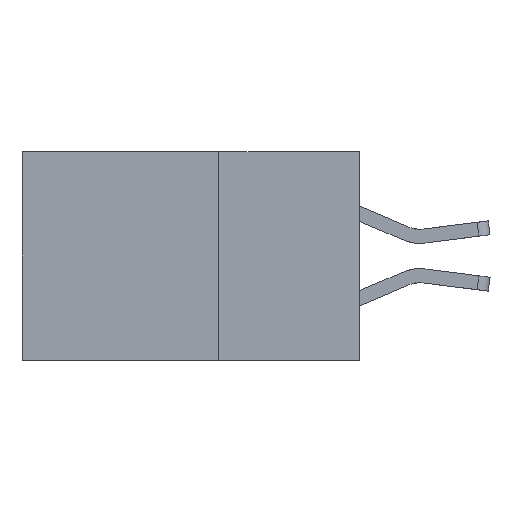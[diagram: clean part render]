
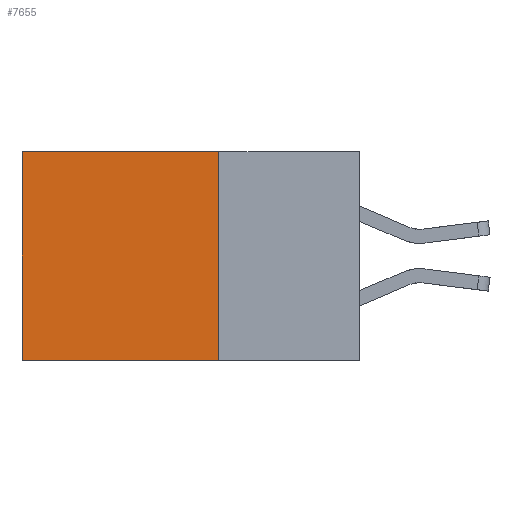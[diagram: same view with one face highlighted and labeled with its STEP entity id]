
A CAD part, left-side view. The second image highlights one B-rep face of the part: STEP entity #7655.
In plain terms, the highlighted planar face has unit normal (-1, 0, 0).
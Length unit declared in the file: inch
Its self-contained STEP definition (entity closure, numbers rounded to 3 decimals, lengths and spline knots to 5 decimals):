
#774 = VECTOR ( 'NONE', #14064, 39.37008 ) ;
#1554 = ORIENTED_EDGE ( 'NONE', *, *, #13683, .T. ) ;
#1603 = CARTESIAN_POINT ( 'NONE',  ( 0.2875, 0.25, 0. ) ) ;
#2073 = VERTEX_POINT ( 'NONE', #15092 ) ;
#2474 = EDGE_LOOP ( 'NONE', ( #10835, #10381, #4373, #1554 ) ) ;
#2613 = EDGE_CURVE ( 'NONE', #10566, #2073, #10315, .T. ) ;
#3414 = FACE_OUTER_BOUND ( 'NONE', #2474, .T. ) ;
#3689 = PLANE ( 'NONE',  #7501 ) ;
#4159 = DIRECTION ( 'NONE',  ( 0., 1., 0. ) ) ;
#4251 = CARTESIAN_POINT ( 'NONE',  ( 0.2875, 0.6, 0. ) ) ;
#4373 = ORIENTED_EDGE ( 'NONE', *, *, #2613, .F. ) ;
#4667 = CARTESIAN_POINT ( 'NONE',  ( 0.2875, 0.25, 0. ) ) ;
#4689 = CARTESIAN_POINT ( 'NONE',  ( 0.2875, 0.25, 0. ) ) ;
#4812 = VERTEX_POINT ( 'NONE', #14345 ) ;
#4959 = VERTEX_POINT ( 'NONE', #4251 ) ;
#6323 = VECTOR ( 'NONE', #14890, 39.37008 ) ;
#6869 = LINE ( 'NONE', #15251, #774 ) ;
#7501 = AXIS2_PLACEMENT_3D ( 'NONE', #4689, #13349, #9535 ) ;
#7655 = ADVANCED_FACE ( 'NONE', ( #3414 ), #3689, .F. ) ;
#8329 = VECTOR ( 'NONE', #14919, 39.37008 ) ;
#9535 = DIRECTION ( 'NONE',  ( 0., 0., -1. ) ) ;
#9717 = VECTOR ( 'NONE', #4159, 39.37008 ) ;
#10255 = EDGE_CURVE ( 'NONE', #2073, #4812, #11887, .T. ) ;
#10315 = LINE ( 'NONE', #1603, #6323 ) ;
#10381 = ORIENTED_EDGE ( 'NONE', *, *, #10255, .F. ) ;
#10566 = VERTEX_POINT ( 'NONE', #4667 ) ;
#10835 = ORIENTED_EDGE ( 'NONE', *, *, #14321, .T. ) ;
#11408 = CARTESIAN_POINT ( 'NONE',  ( 0.2875, 0.25, 0. ) ) ;
#11887 = LINE ( 'NONE', #12975, #8329 ) ;
#12975 = CARTESIAN_POINT ( 'NONE',  ( 0.2875, 0.25, -0.37 ) ) ;
#13276 = LINE ( 'NONE', #11408, #9717 ) ;
#13349 = DIRECTION ( 'NONE',  ( 1., 0., 0. ) ) ;
#13683 = EDGE_CURVE ( 'NONE', #10566, #4959, #13276, .T. ) ;
#14064 = DIRECTION ( 'NONE',  ( 0., 0., -1. ) ) ;
#14321 = EDGE_CURVE ( 'NONE', #4959, #4812, #6869, .T. ) ;
#14345 = CARTESIAN_POINT ( 'NONE',  ( 0.2875, 0.6, -0.37 ) ) ;
#14890 = DIRECTION ( 'NONE',  ( 0., 0., -1. ) ) ;
#14919 = DIRECTION ( 'NONE',  ( 0., 1., 0. ) ) ;
#15092 = CARTESIAN_POINT ( 'NONE',  ( 0.2875, 0.25, -0.37 ) ) ;
#15251 = CARTESIAN_POINT ( 'NONE',  ( 0.2875, 0.6, 0. ) ) ;
